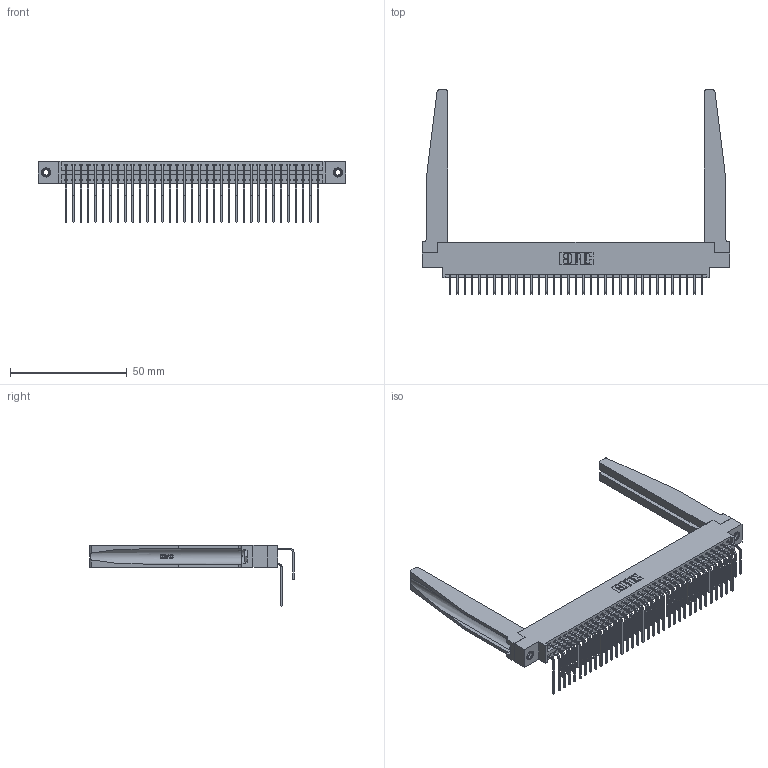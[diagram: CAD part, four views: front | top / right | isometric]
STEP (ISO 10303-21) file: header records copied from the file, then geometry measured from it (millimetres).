
FILE_DESCRIPTION (( 'STEP AP203' ), '1' );
FILE_NAME ('396-070-558-878.STEP', '2019-11-03T11:11:17', ( '' ), ( '' ), 'SwSTEP 2.0', 'SolidWorks 2016', '' );
FILE_SCHEMA (( 'CONFIG_CONTROL_DESIGN' ));
Length unit declared in the file: inch
Products named in the file (6): 345-292-001_558 Tail - 2; 345-250-001_345-250-001-102; 396-070-558-878; 346 Part_0.170 Offset - 0.156 Dia-TH; 345-292-001_558 559 Tail - 1; 346-220-078_345-220-078
Assembly tree (75 placements, depth 2):
  396-070-558-878
    346 Part_0.170 Offset - 0.156 Dia-TH
    345-292-001_558 559 Tail - 1  x35
    345-292-001_558 Tail - 2  x35
    346-220-078_345-220-078  x2
    345-250-001_345-250-001-102  x2
Bounding box: 131.7 x 87.44 x 26.16 mm (x, y, z)
Volume: 19946 mm3; surface area: 26464.7 mm2
Topology: 75 solids, 75 shells, 4140 faces, 12219 edges, 8042 vertices
Faces by surface type: plane 2812, cylinder 1276, bspline 36, cone 12, torus 4
Entity records: 30448 total; most frequent: CARTESIAN_POINT 6018, ORIENTED_EDGE 4790, DIRECTION 4313, EDGE_CURVE 2395, VECTOR 1989, LINE 1989, VERTEX_POINT 1588, AXIS2_PLACEMENT_3D 1162
